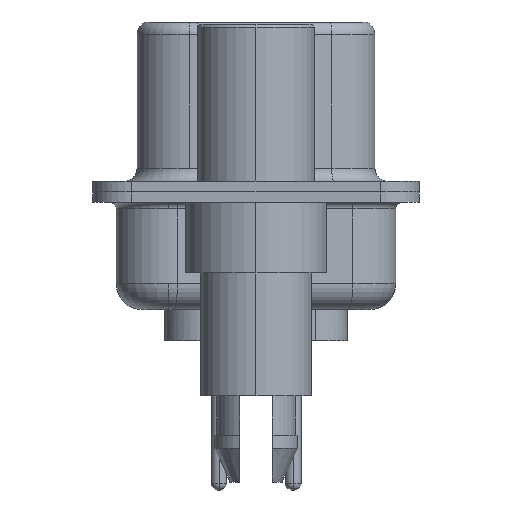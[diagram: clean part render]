
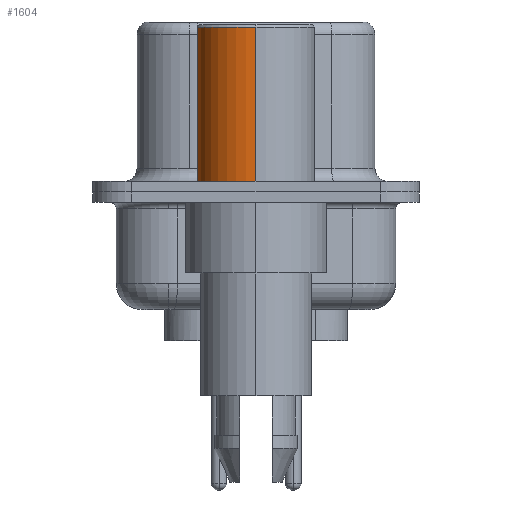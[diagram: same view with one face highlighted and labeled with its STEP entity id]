
A CAD part, left-side view. The second image highlights one B-rep face of the part: STEP entity #1604.
In plain terms, the highlighted cylindrical face has radius 2.25 mm (diameter 4.5 mm), a partial arc.
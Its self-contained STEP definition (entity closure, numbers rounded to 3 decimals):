
#129 = EDGE_CURVE ( 'NONE', #6816, #4076, #6309, .T. ) ;
#372 = DIRECTION ( 'NONE',  ( 1., 0., 0. ) ) ;
#848 = CARTESIAN_POINT ( 'NONE',  ( -2.25, 0., 6.3 ) ) ;
#1224 = AXIS2_PLACEMENT_3D ( 'NONE', #9908, #1682, #372 ) ;
#1604 = ADVANCED_FACE ( 'NONE', ( #11068 ), #15073, .T. ) ;
#1642 = DIRECTION ( 'NONE',  ( 0., 0., 1. ) ) ;
#1682 = DIRECTION ( 'NONE',  ( 0., 0., 1. ) ) ;
#2530 = EDGE_CURVE ( 'NONE', #6250, #16427, #8392, .T. ) ;
#3262 = CARTESIAN_POINT ( 'NONE',  ( 0., 0., 0.581 ) ) ;
#3579 = ORIENTED_EDGE ( 'NONE', *, *, #10356, .F. ) ;
#4076 = VERTEX_POINT ( 'NONE', #16858 ) ;
#4452 = CARTESIAN_POINT ( 'NONE',  ( -2.25, 0., 0.581 ) ) ;
#5003 = CARTESIAN_POINT ( 'NONE',  ( 2.25, 0., 0.581 ) ) ;
#5192 = AXIS2_PLACEMENT_3D ( 'NONE', #10472, #14565, #7921 ) ;
#5905 = DIRECTION ( 'NONE',  ( 0., 0., 1. ) ) ;
#6250 = VERTEX_POINT ( 'NONE', #15675 ) ;
#6309 = LINE ( 'NONE', #5003, #13569 ) ;
#6398 = DIRECTION ( 'NONE',  ( 0., 0., 1. ) ) ;
#6816 = VERTEX_POINT ( 'NONE', #9629 ) ;
#7921 = DIRECTION ( 'NONE',  ( 1., 0., 0. ) ) ;
#8345 = DIRECTION ( 'NONE',  ( 1., 0., 0. ) ) ;
#8392 = LINE ( 'NONE', #4452, #16733 ) ;
#9629 = CARTESIAN_POINT ( 'NONE',  ( 2.25, 0., 0.4 ) ) ;
#9908 = CARTESIAN_POINT ( 'NONE',  ( 0., 0., 6.3 ) ) ;
#10356 = EDGE_CURVE ( 'NONE', #4076, #16427, #17153, .T. ) ;
#10440 = ORIENTED_EDGE ( 'NONE', *, *, #2530, .T. ) ;
#10472 = CARTESIAN_POINT ( 'NONE',  ( 0., 0., 0.4 ) ) ;
#10497 = CIRCLE ( 'NONE', #5192, 2.25 ) ;
#11068 = FACE_OUTER_BOUND ( 'NONE', #15431, .T. ) ;
#11590 = EDGE_CURVE ( 'NONE', #6816, #6250, #10497, .T. ) ;
#11779 = AXIS2_PLACEMENT_3D ( 'NONE', #3262, #5905, #8345 ) ;
#13569 = VECTOR ( 'NONE', #6398, 1000. ) ;
#13839 = ORIENTED_EDGE ( 'NONE', *, *, #11590, .T. ) ;
#14565 = DIRECTION ( 'NONE',  ( 0., 0., 1. ) ) ;
#14834 = ORIENTED_EDGE ( 'NONE', *, *, #129, .F. ) ;
#15073 = CYLINDRICAL_SURFACE ( 'NONE', #11779, 2.25 ) ;
#15431 = EDGE_LOOP ( 'NONE', ( #13839, #10440, #3579, #14834 ) ) ;
#15675 = CARTESIAN_POINT ( 'NONE',  ( -2.25, 0., 0.4 ) ) ;
#16427 = VERTEX_POINT ( 'NONE', #848 ) ;
#16733 = VECTOR ( 'NONE', #1642, 1000. ) ;
#16858 = CARTESIAN_POINT ( 'NONE',  ( 2.25, 0., 6.3 ) ) ;
#17153 = CIRCLE ( 'NONE', #1224, 2.25 ) ;
